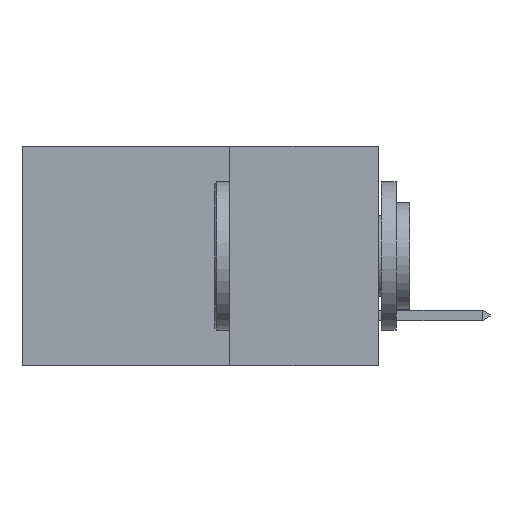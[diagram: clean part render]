
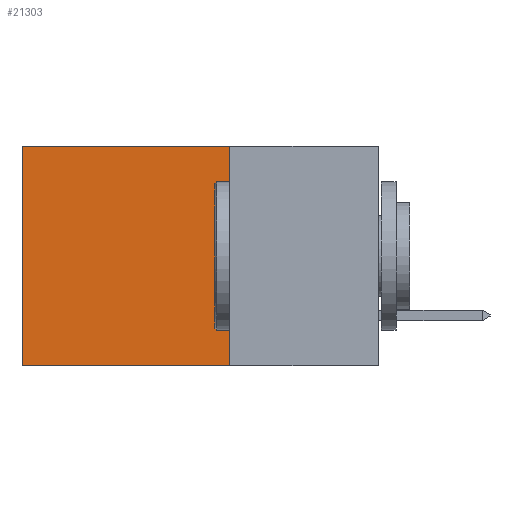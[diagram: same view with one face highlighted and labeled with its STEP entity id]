
A CAD part, left-side view. The second image highlights one B-rep face of the part: STEP entity #21303.
In plain terms, the highlighted planar face has unit normal (-1, 0, 0).
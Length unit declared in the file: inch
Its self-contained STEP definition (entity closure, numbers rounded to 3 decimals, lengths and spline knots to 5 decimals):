
#532 = CARTESIAN_POINT ( 'NONE',  ( 0.2615, 0.25, -0.37 ) ) ;
#1739 = CARTESIAN_POINT ( 'NONE',  ( 0.2615, 0.25, -0.37 ) ) ;
#2590 = LINE ( 'NONE', #8609, #24081 ) ;
#2714 = VERTEX_POINT ( 'NONE', #25349 ) ;
#2738 = EDGE_CURVE ( 'NONE', #18545, #2714, #26337, .T. ) ;
#2828 = VECTOR ( 'NONE', #3901, 39.37008 ) ;
#3901 = DIRECTION ( 'NONE',  ( 0., 1., 0. ) ) ;
#4337 = VECTOR ( 'NONE', #23513, 39.37008 ) ;
#4471 = DIRECTION ( 'NONE',  ( 0., 0., -1. ) ) ;
#6392 = VERTEX_POINT ( 'NONE', #532 ) ;
#6466 = ORIENTED_EDGE ( 'NONE', *, *, #2738, .T. ) ;
#7591 = ORIENTED_EDGE ( 'NONE', *, *, #10745, .T. ) ;
#8473 = CARTESIAN_POINT ( 'NONE',  ( 0.2615, 0.25, -0.37 ) ) ;
#8609 = CARTESIAN_POINT ( 'NONE',  ( 0.2615, 0.6, -0.37 ) ) ;
#8662 = CARTESIAN_POINT ( 'NONE',  ( 0.2615, 0.25, -0.37 ) ) ;
#10589 = DIRECTION ( 'NONE',  ( 0., 0., -1. ) ) ;
#10745 = EDGE_CURVE ( 'NONE', #2714, #24119, #2590, .T. ) ;
#10776 = DIRECTION ( 'NONE',  ( 0., 0., -1. ) ) ;
#12570 = EDGE_CURVE ( 'NONE', #18545, #6392, #26486, .T. ) ;
#12749 = PLANE ( 'NONE',  #15243 ) ;
#14002 = LINE ( 'NONE', #1739, #2828 ) ;
#15243 = AXIS2_PLACEMENT_3D ( 'NONE', #8662, #23122, #10776 ) ;
#18545 = VERTEX_POINT ( 'NONE', #26253 ) ;
#18652 = EDGE_CURVE ( 'NONE', #6392, #24119, #14002, .T. ) ;
#19569 = ORIENTED_EDGE ( 'NONE', *, *, #18652, .F. ) ;
#20966 = ORIENTED_EDGE ( 'NONE', *, *, #12570, .F. ) ;
#21303 = ADVANCED_FACE ( 'NONE', ( #24460 ), #12749, .F. ) ;
#23122 = DIRECTION ( 'NONE',  ( 1., 0., 0. ) ) ;
#23405 = CARTESIAN_POINT ( 'NONE',  ( 0.2615, 0.6, -0.37 ) ) ;
#23513 = DIRECTION ( 'NONE',  ( 0., 1., 0. ) ) ;
#23644 = VECTOR ( 'NONE', #10589, 39.37008 ) ;
#23889 = CARTESIAN_POINT ( 'NONE',  ( 0.2615, 0.25, 0. ) ) ;
#24081 = VECTOR ( 'NONE', #4471, 39.37008 ) ;
#24119 = VERTEX_POINT ( 'NONE', #23405 ) ;
#24460 = FACE_OUTER_BOUND ( 'NONE', #25688, .T. ) ;
#25349 = CARTESIAN_POINT ( 'NONE',  ( 0.2615, 0.6, 0. ) ) ;
#25688 = EDGE_LOOP ( 'NONE', ( #7591, #19569, #20966, #6466 ) ) ;
#26253 = CARTESIAN_POINT ( 'NONE',  ( 0.2615, 0.25, 0. ) ) ;
#26337 = LINE ( 'NONE', #23889, #4337 ) ;
#26486 = LINE ( 'NONE', #8473, #23644 ) ;
